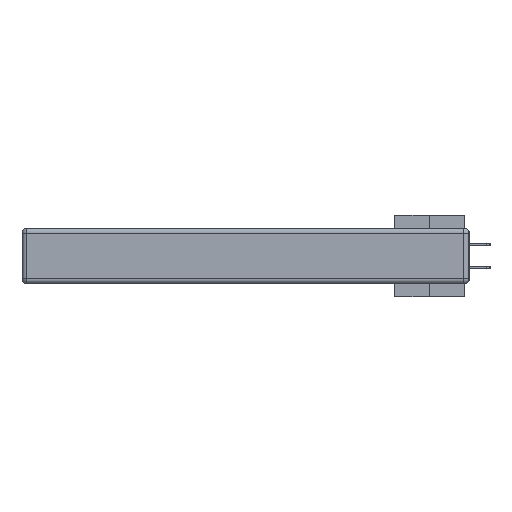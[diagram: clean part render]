
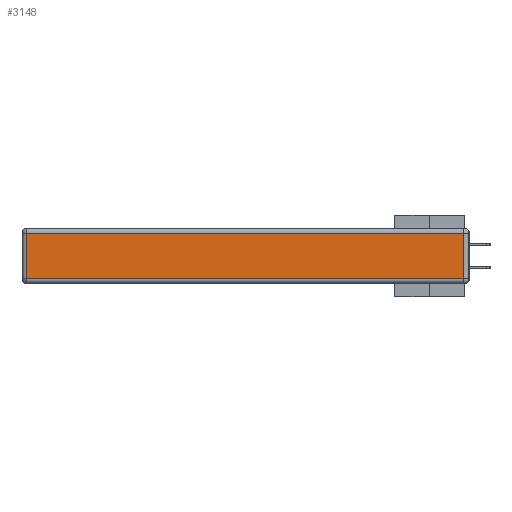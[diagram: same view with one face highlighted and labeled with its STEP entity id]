
A CAD part, left-side view. The second image highlights one B-rep face of the part: STEP entity #3148.
In plain terms, the highlighted planar face has unit normal (-1, 0, 0).
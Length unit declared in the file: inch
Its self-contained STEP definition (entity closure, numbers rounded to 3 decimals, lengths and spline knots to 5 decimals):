
#893 = PLANE ( 'NONE',  #30578 ) ;
#1291 = VECTOR ( 'NONE', #36834, 39.37008 ) ;
#1790 = EDGE_CURVE ( 'NONE', #21289, #26304, #25897, .T. ) ;
#2703 = EDGE_CURVE ( 'NONE', #30382, #21289, #3803, .T. ) ;
#3148 = ADVANCED_FACE ( 'NONE', ( #25026 ), #893, .T. ) ;
#3803 = LINE ( 'NONE', #13622, #32190 ) ;
#4764 = CARTESIAN_POINT ( 'NONE',  ( 0., 0., -0.343 ) ) ;
#7306 = CARTESIAN_POINT ( 'NONE',  ( 0., 2.75, -0.03 ) ) ;
#7421 = VERTEX_POINT ( 'NONE', #16457 ) ;
#10231 = ORIENTED_EDGE ( 'NONE', *, *, #1790, .T. ) ;
#11083 = DIRECTION ( 'NONE',  ( 0., 1., 0. ) ) ;
#13245 = CARTESIAN_POINT ( 'NONE',  ( 0., 2.72, -0.03 ) ) ;
#13622 = CARTESIAN_POINT ( 'NONE',  ( 0., 2.72, -0.343 ) ) ;
#14444 = ORIENTED_EDGE ( 'NONE', *, *, #42154, .T. ) ;
#15839 = VECTOR ( 'NONE', #42920, 39.37008 ) ;
#16457 = CARTESIAN_POINT ( 'NONE',  ( 0., 0.03, -0.03 ) ) ;
#19929 = CARTESIAN_POINT ( 'NONE',  ( 0., 0., -0.313 ) ) ;
#21024 = ORIENTED_EDGE ( 'NONE', *, *, #2703, .T. ) ;
#21289 = VERTEX_POINT ( 'NONE', #23285 ) ;
#23285 = CARTESIAN_POINT ( 'NONE',  ( 0., 2.72, -0.313 ) ) ;
#25026 = FACE_OUTER_BOUND ( 'NONE', #47830, .T. ) ;
#25410 = CARTESIAN_POINT ( 'NONE',  ( 0., 0.03, -0.343 ) ) ;
#25897 = LINE ( 'NONE', #19929, #15839 ) ;
#26304 = VERTEX_POINT ( 'NONE', #34983 ) ;
#28576 = VECTOR ( 'NONE', #11083, 39.37008 ) ;
#30204 = DIRECTION ( 'NONE',  ( 0., 0., 1. ) ) ;
#30382 = VERTEX_POINT ( 'NONE', #13245 ) ;
#30578 = AXIS2_PLACEMENT_3D ( 'NONE', #4764, #40317, #30204 ) ;
#32190 = VECTOR ( 'NONE', #47532, 39.37008 ) ;
#34983 = CARTESIAN_POINT ( 'NONE',  ( 0., 0.03, -0.313 ) ) ;
#36834 = DIRECTION ( 'NONE',  ( 0., 0., 1. ) ) ;
#38267 = EDGE_CURVE ( 'NONE', #26304, #7421, #48119, .T. ) ;
#38293 = ORIENTED_EDGE ( 'NONE', *, *, #38267, .T. ) ;
#40317 = DIRECTION ( 'NONE',  ( -1., 0., 0. ) ) ;
#42154 = EDGE_CURVE ( 'NONE', #7421, #30382, #42744, .T. ) ;
#42744 = LINE ( 'NONE', #7306, #28576 ) ;
#42920 = DIRECTION ( 'NONE',  ( 0., -1., 0. ) ) ;
#47532 = DIRECTION ( 'NONE',  ( 0., 0., -1. ) ) ;
#47830 = EDGE_LOOP ( 'NONE', ( #10231, #38293, #14444, #21024 ) ) ;
#48119 = LINE ( 'NONE', #25410, #1291 ) ;
